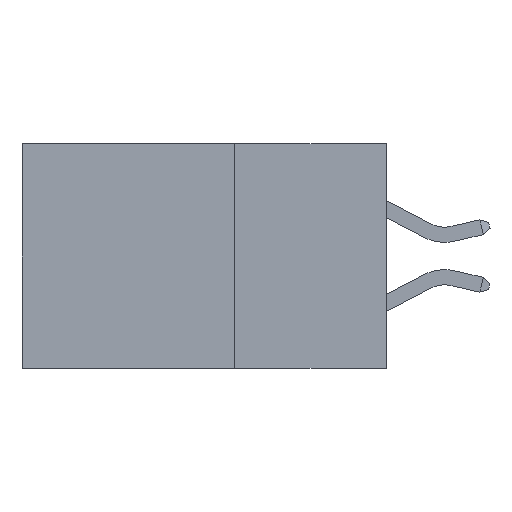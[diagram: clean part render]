
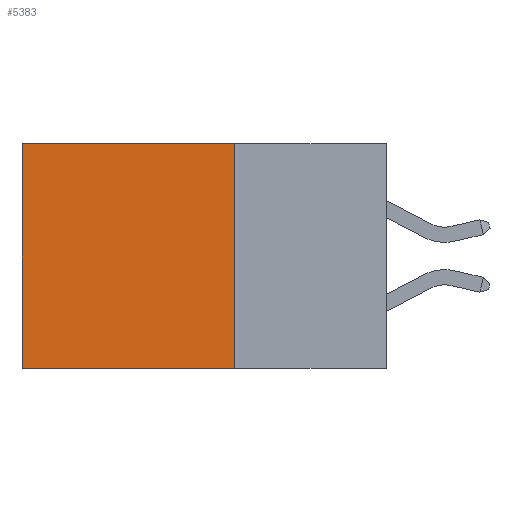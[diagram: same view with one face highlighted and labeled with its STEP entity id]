
A CAD part, left-side view. The second image highlights one B-rep face of the part: STEP entity #5383.
In plain terms, the highlighted planar face has unit normal (-1, 0, 0).
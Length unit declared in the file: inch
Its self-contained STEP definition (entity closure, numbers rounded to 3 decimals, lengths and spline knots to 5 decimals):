
#20 = VERTEX_POINT ( 'NONE', #5170 ) ;
#34 = CARTESIAN_POINT ( 'NONE',  ( 0.2615, 0.25, -0.37 ) ) ;
#164 = LINE ( 'NONE', #1284, #10790 ) ;
#399 = LINE ( 'NONE', #5995, #10728 ) ;
#1284 = CARTESIAN_POINT ( 'NONE',  ( 0.2615, 0.25, 0. ) ) ;
#1457 = VERTEX_POINT ( 'NONE', #10121 ) ;
#1939 = PLANE ( 'NONE',  #9906 ) ;
#2039 = VECTOR ( 'NONE', #6962, 39.37008 ) ;
#2327 = CARTESIAN_POINT ( 'NONE',  ( 0.2615, 0.25, -0.37 ) ) ;
#3127 = EDGE_LOOP ( 'NONE', ( #5202, #4833, #8535, #4902 ) ) ;
#3776 = VERTEX_POINT ( 'NONE', #11697 ) ;
#3847 = DIRECTION ( 'NONE',  ( 1., 0., 0. ) ) ;
#4113 = DIRECTION ( 'NONE',  ( 0., 0., -1. ) ) ;
#4226 = VERTEX_POINT ( 'NONE', #7585 ) ;
#4336 = EDGE_CURVE ( 'NONE', #3776, #20, #399, .T. ) ;
#4833 = ORIENTED_EDGE ( 'NONE', *, *, #6719, .F. ) ;
#4869 = FACE_OUTER_BOUND ( 'NONE', #3127, .T. ) ;
#4901 = VECTOR ( 'NONE', #4113, 39.37008 ) ;
#4902 = ORIENTED_EDGE ( 'NONE', *, *, #11759, .T. ) ;
#5053 = DIRECTION ( 'NONE',  ( 0., 1., 0. ) ) ;
#5170 = CARTESIAN_POINT ( 'NONE',  ( 0.2615, 0.6, -0.37 ) ) ;
#5202 = ORIENTED_EDGE ( 'NONE', *, *, #4336, .T. ) ;
#5383 = ADVANCED_FACE ( 'NONE', ( #4869 ), #1939, .F. ) ;
#5995 = CARTESIAN_POINT ( 'NONE',  ( 0.2615, 0.6, -0.37 ) ) ;
#6719 = EDGE_CURVE ( 'NONE', #1457, #20, #8034, .T. ) ;
#6962 = DIRECTION ( 'NONE',  ( 0., 1., 0. ) ) ;
#7108 = EDGE_CURVE ( 'NONE', #4226, #1457, #10742, .T. ) ;
#7585 = CARTESIAN_POINT ( 'NONE',  ( 0.2615, 0.25, 0. ) ) ;
#8013 = DIRECTION ( 'NONE',  ( 0., 0., -1. ) ) ;
#8034 = LINE ( 'NONE', #2327, #2039 ) ;
#8535 = ORIENTED_EDGE ( 'NONE', *, *, #7108, .F. ) ;
#8728 = DIRECTION ( 'NONE',  ( 0., 0., -1. ) ) ;
#9906 = AXIS2_PLACEMENT_3D ( 'NONE', #34, #3847, #8728 ) ;
#9994 = CARTESIAN_POINT ( 'NONE',  ( 0.2615, 0.25, -0.37 ) ) ;
#10121 = CARTESIAN_POINT ( 'NONE',  ( 0.2615, 0.25, -0.37 ) ) ;
#10728 = VECTOR ( 'NONE', #8013, 39.37008 ) ;
#10742 = LINE ( 'NONE', #9994, #4901 ) ;
#10790 = VECTOR ( 'NONE', #5053, 39.37008 ) ;
#11697 = CARTESIAN_POINT ( 'NONE',  ( 0.2615, 0.6, 0. ) ) ;
#11759 = EDGE_CURVE ( 'NONE', #4226, #3776, #164, .T. ) ;
